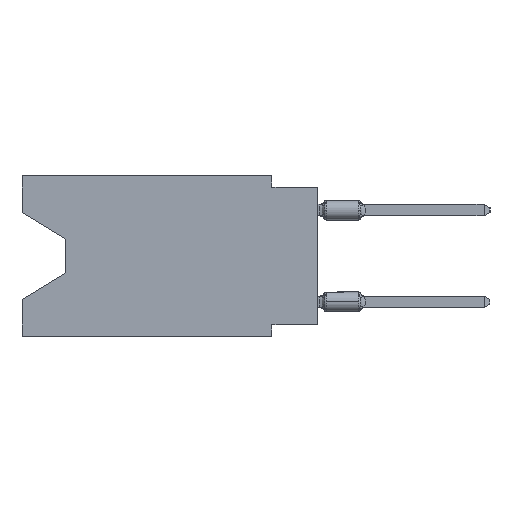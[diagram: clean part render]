
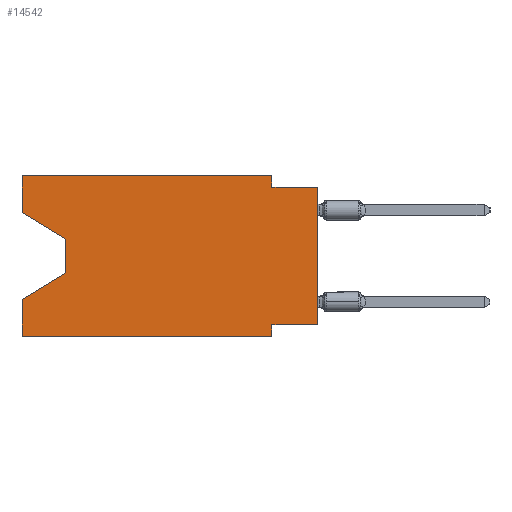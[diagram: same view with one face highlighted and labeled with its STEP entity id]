
A CAD part, left-side view. The second image highlights one B-rep face of the part: STEP entity #14542.
In plain terms, the highlighted planar face has unit normal (-1, 0, 0).
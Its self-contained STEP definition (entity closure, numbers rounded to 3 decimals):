
#137 = EDGE_CURVE ( 'NONE', #9090, #16618, #146, .T. ) ;
#146 = LINE ( 'NONE', #8118, #18615 ) ;
#312 = EDGE_LOOP ( 'NONE', ( #17500, #12235, #16804, #23778, #6455, #13715, #10462, #20322, #13904, #3475, #15149, #8001 ) ) ;
#968 = DIRECTION ( 'NONE',  ( 0., -1., 0. ) ) ;
#1525 = VERTEX_POINT ( 'NONE', #20606 ) ;
#1534 = LINE ( 'NONE', #12796, #11709 ) ;
#1758 = LINE ( 'NONE', #9391, #13386 ) ;
#1953 = CARTESIAN_POINT ( 'NONE',  ( 0., 0., -0.635 ) ) ;
#2481 = LINE ( 'NONE', #14109, #4548 ) ;
#2563 = CARTESIAN_POINT ( 'NONE',  ( 0., 16.383, -2.038 ) ) ;
#3171 = CARTESIAN_POINT ( 'NONE',  ( 0., 13.97, -3.505 ) ) ;
#3287 = DIRECTION ( 'NONE',  ( 0., 0., -1. ) ) ;
#3385 = VECTOR ( 'NONE', #7959, 1000. ) ;
#3475 = ORIENTED_EDGE ( 'NONE', *, *, #4522, .F. ) ;
#3757 = VECTOR ( 'NONE', #7083, 1000. ) ;
#3957 = LINE ( 'NONE', #1953, #17239 ) ;
#4522 = EDGE_CURVE ( 'NONE', #1525, #22574, #2481, .T. ) ;
#4548 = VECTOR ( 'NONE', #21724, 1000. ) ;
#4658 = EDGE_CURVE ( 'NONE', #9090, #6112, #22198, .T. ) ;
#4914 = VECTOR ( 'NONE', #18798, 1000. ) ;
#5561 = CARTESIAN_POINT ( 'NONE',  ( 0., 16.383, -2.038 ) ) ;
#5617 = EDGE_CURVE ( 'NONE', #14255, #6590, #20801, .T. ) ;
#5659 = CARTESIAN_POINT ( 'NONE',  ( 0., 16.383, 0. ) ) ;
#6112 = VERTEX_POINT ( 'NONE', #19707 ) ;
#6141 = CARTESIAN_POINT ( 'NONE',  ( 0., 13.97, -5.385 ) ) ;
#6191 = CARTESIAN_POINT ( 'NONE',  ( 0., 0., -0.635 ) ) ;
#6198 = CARTESIAN_POINT ( 'NONE',  ( 0., 13.97, -3.505 ) ) ;
#6455 = ORIENTED_EDGE ( 'NONE', *, *, #137, .T. ) ;
#6590 = VERTEX_POINT ( 'NONE', #3171 ) ;
#6641 = DIRECTION ( 'NONE',  ( 0., 0.855, -0.519 ) ) ;
#7083 = DIRECTION ( 'NONE',  ( 0., 0., 1. ) ) ;
#7209 = CARTESIAN_POINT ( 'NONE',  ( 0., 16.383, 0. ) ) ;
#7959 = DIRECTION ( 'NONE',  ( 0., 0., -1. ) ) ;
#8001 = ORIENTED_EDGE ( 'NONE', *, *, #14793, .F. ) ;
#8118 = CARTESIAN_POINT ( 'NONE',  ( 0., 16.383, -8.89 ) ) ;
#8681 = EDGE_CURVE ( 'NONE', #20420, #6112, #18233, .T. ) ;
#9090 = VERTEX_POINT ( 'NONE', #12111 ) ;
#9167 = DIRECTION ( 'NONE',  ( 0., 0., 1. ) ) ;
#9391 = CARTESIAN_POINT ( 'NONE',  ( 0., 2.54, -8.89 ) ) ;
#9593 = DIRECTION ( 'NONE',  ( 0., -1., 0. ) ) ;
#9790 = CARTESIAN_POINT ( 'NONE',  ( 0., 16.383, 0. ) ) ;
#10011 = VECTOR ( 'NONE', #6641, 1000. ) ;
#10199 = LINE ( 'NONE', #6198, #3385 ) ;
#10330 = DIRECTION ( 'NONE',  ( 0., -1., 0. ) ) ;
#10462 = ORIENTED_EDGE ( 'NONE', *, *, #22989, .F. ) ;
#10867 = CARTESIAN_POINT ( 'NONE',  ( 0., 16.383, 0. ) ) ;
#10883 = VERTEX_POINT ( 'NONE', #24144 ) ;
#11168 = DIRECTION ( 'NONE',  ( 1., 0., 0. ) ) ;
#11560 = CARTESIAN_POINT ( 'NONE',  ( 0., 2.54, -0.635 ) ) ;
#11709 = VECTOR ( 'NONE', #9167, 1000. ) ;
#11900 = LINE ( 'NONE', #12142, #22219 ) ;
#11958 = LINE ( 'NONE', #17809, #12852 ) ;
#11976 = VERTEX_POINT ( 'NONE', #6191 ) ;
#12111 = CARTESIAN_POINT ( 'NONE',  ( 0., 16.383, -8.89 ) ) ;
#12142 = CARTESIAN_POINT ( 'NONE',  ( 0., 0., -8.255 ) ) ;
#12235 = ORIENTED_EDGE ( 'NONE', *, *, #20890, .T. ) ;
#12796 = CARTESIAN_POINT ( 'NONE',  ( 0., 0., 0. ) ) ;
#12852 = VECTOR ( 'NONE', #10330, 1000. ) ;
#13386 = VECTOR ( 'NONE', #15398, 1000. ) ;
#13715 = ORIENTED_EDGE ( 'NONE', *, *, #21761, .F. ) ;
#13904 = ORIENTED_EDGE ( 'NONE', *, *, #23616, .F. ) ;
#14109 = CARTESIAN_POINT ( 'NONE',  ( 0., 2.54, 0. ) ) ;
#14255 = VERTEX_POINT ( 'NONE', #2563 ) ;
#14542 = ADVANCED_FACE ( 'NONE', ( #14792 ), #22519, .F. ) ;
#14792 = FACE_OUTER_BOUND ( 'NONE', #312, .T. ) ;
#14793 = EDGE_CURVE ( 'NONE', #14255, #21105, #23972, .T. ) ;
#15149 = ORIENTED_EDGE ( 'NONE', *, *, #23881, .F. ) ;
#15332 = CARTESIAN_POINT ( 'NONE',  ( 0., 2.54, -8.89 ) ) ;
#15398 = DIRECTION ( 'NONE',  ( 0., 0., -1. ) ) ;
#15838 = EDGE_CURVE ( 'NONE', #20533, #11976, #1534, .T. ) ;
#16604 = DIRECTION ( 'NONE',  ( 0., 0., 1. ) ) ;
#16618 = VERTEX_POINT ( 'NONE', #15332 ) ;
#16804 = ORIENTED_EDGE ( 'NONE', *, *, #8681, .T. ) ;
#16824 = AXIS2_PLACEMENT_3D ( 'NONE', #5659, #11168, #3287 ) ;
#17239 = VECTOR ( 'NONE', #9593, 1000. ) ;
#17500 = ORIENTED_EDGE ( 'NONE', *, *, #5617, .T. ) ;
#17809 = CARTESIAN_POINT ( 'NONE',  ( 0., 16.383, 0. ) ) ;
#18233 = LINE ( 'NONE', #20110, #10011 ) ;
#18615 = VECTOR ( 'NONE', #968, 1000. ) ;
#18798 = DIRECTION ( 'NONE',  ( 0., -0.855, -0.519 ) ) ;
#19248 = CARTESIAN_POINT ( 'NONE',  ( 0., 0., -8.255 ) ) ;
#19707 = CARTESIAN_POINT ( 'NONE',  ( 0., 16.383, -6.852 ) ) ;
#20110 = CARTESIAN_POINT ( 'NONE',  ( 0., 13.97, -5.385 ) ) ;
#20322 = ORIENTED_EDGE ( 'NONE', *, *, #15838, .T. ) ;
#20420 = VERTEX_POINT ( 'NONE', #6141 ) ;
#20533 = VERTEX_POINT ( 'NONE', #19248 ) ;
#20606 = CARTESIAN_POINT ( 'NONE',  ( 0., 2.54, 0. ) ) ;
#20801 = LINE ( 'NONE', #5561, #4914 ) ;
#20890 = EDGE_CURVE ( 'NONE', #6590, #20420, #10199, .T. ) ;
#21105 = VERTEX_POINT ( 'NONE', #9790 ) ;
#21724 = DIRECTION ( 'NONE',  ( 0., 0., -1. ) ) ;
#21761 = EDGE_CURVE ( 'NONE', #10883, #16618, #1758, .T. ) ;
#22027 = VECTOR ( 'NONE', #16604, 1000. ) ;
#22198 = LINE ( 'NONE', #7209, #3757 ) ;
#22219 = VECTOR ( 'NONE', #23382, 1000. ) ;
#22519 = PLANE ( 'NONE',  #16824 ) ;
#22574 = VERTEX_POINT ( 'NONE', #11560 ) ;
#22989 = EDGE_CURVE ( 'NONE', #20533, #10883, #11900, .T. ) ;
#23382 = DIRECTION ( 'NONE',  ( 0., 1., 0. ) ) ;
#23616 = EDGE_CURVE ( 'NONE', #22574, #11976, #3957, .T. ) ;
#23778 = ORIENTED_EDGE ( 'NONE', *, *, #4658, .F. ) ;
#23881 = EDGE_CURVE ( 'NONE', #21105, #1525, #11958, .T. ) ;
#23972 = LINE ( 'NONE', #10867, #22027 ) ;
#24144 = CARTESIAN_POINT ( 'NONE',  ( 0., 2.54, -8.255 ) ) ;
